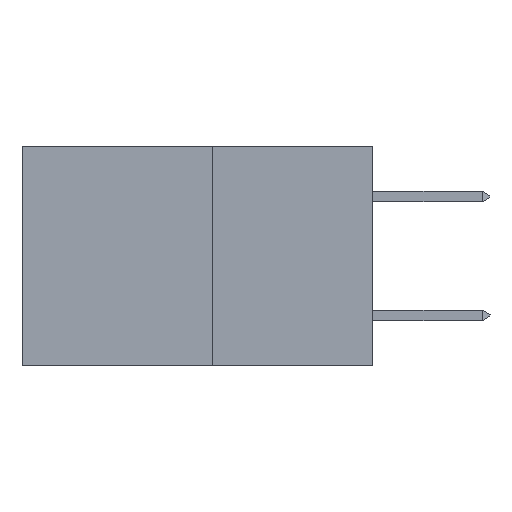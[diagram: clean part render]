
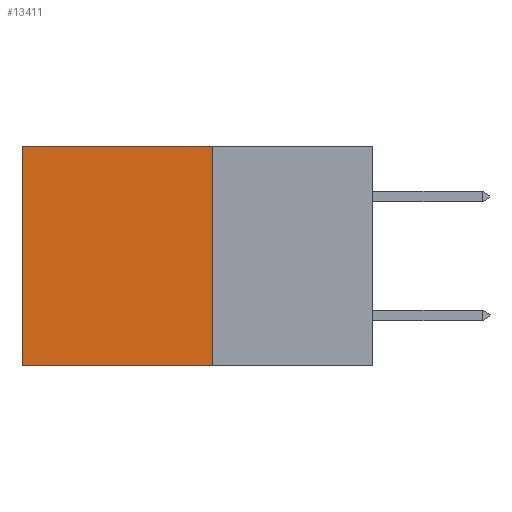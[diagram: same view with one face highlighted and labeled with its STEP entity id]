
A CAD part, left-side view. The second image highlights one B-rep face of the part: STEP entity #13411.
In plain terms, the highlighted planar face has unit normal (-1, 0, 0).
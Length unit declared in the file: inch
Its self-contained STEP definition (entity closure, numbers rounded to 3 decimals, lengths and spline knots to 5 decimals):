
#201 = FACE_OUTER_BOUND ( 'NONE', #9321, .T. ) ;
#767 = VERTEX_POINT ( 'NONE', #14061 ) ;
#1024 = EDGE_CURVE ( 'NONE', #767, #10526, #12262, .T. ) ;
#1466 = CARTESIAN_POINT ( 'NONE',  ( 0.277, 0.59, -0.37 ) ) ;
#3100 = VERTEX_POINT ( 'NONE', #6435 ) ;
#3250 = CARTESIAN_POINT ( 'NONE',  ( 0.277, 0.27, -0.37 ) ) ;
#4402 = DIRECTION ( 'NONE',  ( 0., 0., -1. ) ) ;
#5211 = DIRECTION ( 'NONE',  ( 0., 0., -1. ) ) ;
#5303 = LINE ( 'NONE', #13756, #8208 ) ;
#5737 = LINE ( 'NONE', #1466, #8947 ) ;
#5768 = CARTESIAN_POINT ( 'NONE',  ( 0.277, 0.27, 0. ) ) ;
#6153 = EDGE_CURVE ( 'NONE', #10526, #3100, #5737, .T. ) ;
#6435 = CARTESIAN_POINT ( 'NONE',  ( 0.277, 0.59, -0.37 ) ) ;
#6539 = VERTEX_POINT ( 'NONE', #13330 ) ;
#6546 = DIRECTION ( 'NONE',  ( 0., 0., -1. ) ) ;
#6617 = VECTOR ( 'NONE', #9558, 39.37008 ) ;
#8115 = DIRECTION ( 'NONE',  ( 0., 1., 0. ) ) ;
#8208 = VECTOR ( 'NONE', #5211, 39.37008 ) ;
#8863 = AXIS2_PLACEMENT_3D ( 'NONE', #3250, #10920, #4402 ) ;
#8947 = VECTOR ( 'NONE', #6546, 39.37008 ) ;
#8977 = VECTOR ( 'NONE', #8115, 39.37008 ) ;
#9321 = EDGE_LOOP ( 'NONE', ( #11038, #11158, #11169, #11230 ) ) ;
#9558 = DIRECTION ( 'NONE',  ( 0., 1., 0. ) ) ;
#10526 = VERTEX_POINT ( 'NONE', #13357 ) ;
#10848 = EDGE_CURVE ( 'NONE', #767, #6539, #5303, .T. ) ;
#10920 = DIRECTION ( 'NONE',  ( 1., 0., 0. ) ) ;
#11038 = ORIENTED_EDGE ( 'NONE', *, *, #6153, .T. ) ;
#11158 = ORIENTED_EDGE ( 'NONE', *, *, #12883, .F. ) ;
#11169 = ORIENTED_EDGE ( 'NONE', *, *, #10848, .F. ) ;
#11230 = ORIENTED_EDGE ( 'NONE', *, *, #1024, .T. ) ;
#11827 = LINE ( 'NONE', #12354, #8977 ) ;
#12262 = LINE ( 'NONE', #5768, #6617 ) ;
#12354 = CARTESIAN_POINT ( 'NONE',  ( 0.277, 0.27, -0.37 ) ) ;
#12883 = EDGE_CURVE ( 'NONE', #6539, #3100, #11827, .T. ) ;
#13330 = CARTESIAN_POINT ( 'NONE',  ( 0.277, 0.27, -0.37 ) ) ;
#13357 = CARTESIAN_POINT ( 'NONE',  ( 0.277, 0.59, 0. ) ) ;
#13411 = ADVANCED_FACE ( 'NONE', ( #201 ), #13999, .F. ) ;
#13756 = CARTESIAN_POINT ( 'NONE',  ( 0.277, 0.27, -0.37 ) ) ;
#13999 = PLANE ( 'NONE',  #8863 ) ;
#14061 = CARTESIAN_POINT ( 'NONE',  ( 0.277, 0.27, 0. ) ) ;
